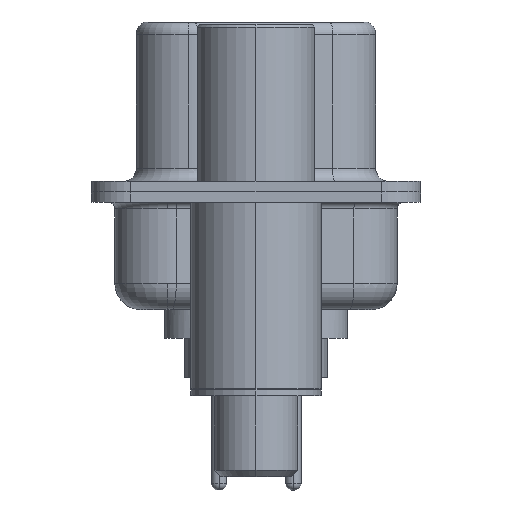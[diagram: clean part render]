
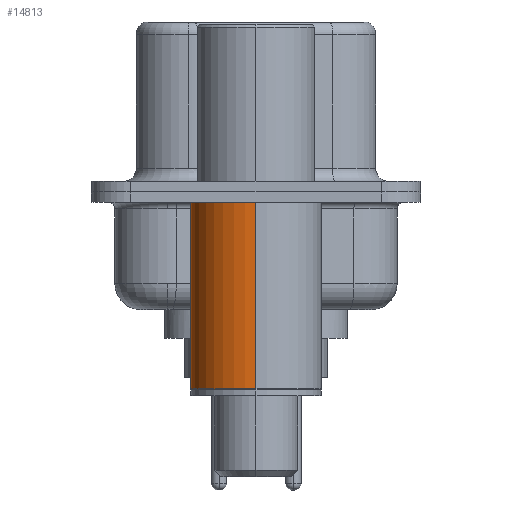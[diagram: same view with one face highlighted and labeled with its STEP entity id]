
A CAD part, left-side view. The second image highlights one B-rep face of the part: STEP entity #14813.
In plain terms, the highlighted cylindrical face has radius 2.5 mm (diameter 5 mm), a partial arc.
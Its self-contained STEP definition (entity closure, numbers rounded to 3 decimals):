
#223 = CYLINDRICAL_SURFACE ( 'NONE', #1801, 2.5 ) ;
#754 = ORIENTED_EDGE ( 'NONE', *, *, #17045, .F. ) ;
#1225 = DIRECTION ( 'NONE',  ( 1., 0., 0. ) ) ;
#1394 = DIRECTION ( 'NONE',  ( 0., 0., 1. ) ) ;
#1751 = CARTESIAN_POINT ( 'NONE',  ( -2.5, 0., -0.4 ) ) ;
#1801 = AXIS2_PLACEMENT_3D ( 'NONE', #10540, #8977, #1225 ) ;
#1886 = CARTESIAN_POINT ( 'NONE',  ( 2.5, 0., -0.4 ) ) ;
#3007 = ORIENTED_EDGE ( 'NONE', *, *, #18780, .T. ) ;
#3170 = AXIS2_PLACEMENT_3D ( 'NONE', #18381, #9017, #19935 ) ;
#5258 = DIRECTION ( 'NONE',  ( 0., 0., 1. ) ) ;
#6113 = VERTEX_POINT ( 'NONE', #1886 ) ;
#7393 = VERTEX_POINT ( 'NONE', #16950 ) ;
#7446 = VECTOR ( 'NONE', #8338, 1000. ) ;
#7937 = LINE ( 'NONE', #19293, #7446 ) ;
#8338 = DIRECTION ( 'NONE',  ( 0., 0., 1. ) ) ;
#8485 = FACE_OUTER_BOUND ( 'NONE', #10648, .T. ) ;
#8745 = CARTESIAN_POINT ( 'NONE',  ( 2.5, 0., -7.525 ) ) ;
#8977 = DIRECTION ( 'NONE',  ( 0., 0., 1. ) ) ;
#9017 = DIRECTION ( 'NONE',  ( 0., 0., 1. ) ) ;
#10264 = LINE ( 'NONE', #12319, #14926 ) ;
#10443 = VERTEX_POINT ( 'NONE', #1751 ) ;
#10540 = CARTESIAN_POINT ( 'NONE',  ( 0., 0., 0.581 ) ) ;
#10648 = EDGE_LOOP ( 'NONE', ( #12544, #3007, #13256, #754 ) ) ;
#10764 = AXIS2_PLACEMENT_3D ( 'NONE', #14635, #5258, #16214 ) ;
#12319 = CARTESIAN_POINT ( 'NONE',  ( -2.5, 0., 0.581 ) ) ;
#12544 = ORIENTED_EDGE ( 'NONE', *, *, #12734, .T. ) ;
#12734 = EDGE_CURVE ( 'NONE', #17202, #7393, #14829, .T. ) ;
#13256 = ORIENTED_EDGE ( 'NONE', *, *, #13473, .F. ) ;
#13473 = EDGE_CURVE ( 'NONE', #6113, #10443, #19681, .T. ) ;
#14635 = CARTESIAN_POINT ( 'NONE',  ( 0., 0., -0.4 ) ) ;
#14813 = ADVANCED_FACE ( 'NONE', ( #8485 ), #223, .T. ) ;
#14829 = CIRCLE ( 'NONE', #3170, 2.5 ) ;
#14926 = VECTOR ( 'NONE', #1394, 1000. ) ;
#16214 = DIRECTION ( 'NONE',  ( 1., 0., 0. ) ) ;
#16950 = CARTESIAN_POINT ( 'NONE',  ( -2.5, 0., -7.525 ) ) ;
#17045 = EDGE_CURVE ( 'NONE', #17202, #6113, #7937, .T. ) ;
#17202 = VERTEX_POINT ( 'NONE', #8745 ) ;
#18381 = CARTESIAN_POINT ( 'NONE',  ( 0., 0., -7.525 ) ) ;
#18780 = EDGE_CURVE ( 'NONE', #7393, #10443, #10264, .T. ) ;
#19293 = CARTESIAN_POINT ( 'NONE',  ( 2.5, 0., 0.581 ) ) ;
#19681 = CIRCLE ( 'NONE', #10764, 2.5 ) ;
#19935 = DIRECTION ( 'NONE',  ( 1., 0., 0. ) ) ;
